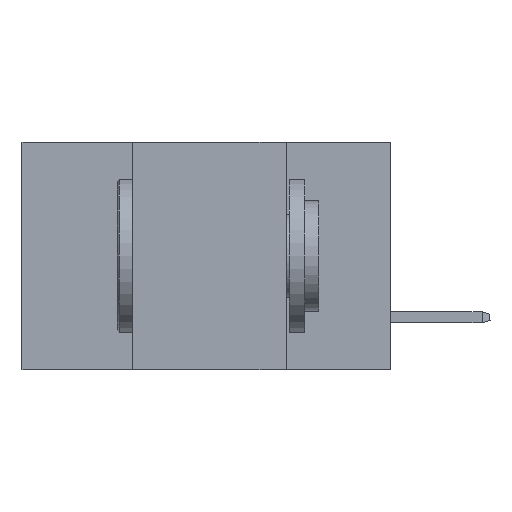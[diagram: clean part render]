
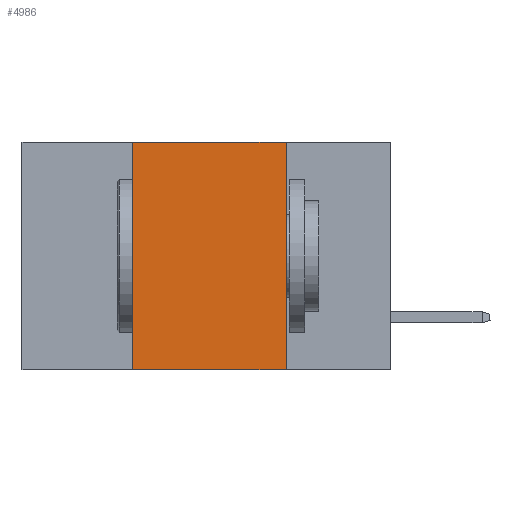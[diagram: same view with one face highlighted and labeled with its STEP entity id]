
A CAD part, left-side view. The second image highlights one B-rep face of the part: STEP entity #4986.
In plain terms, the highlighted planar face has unit normal (-1, 0, 0).
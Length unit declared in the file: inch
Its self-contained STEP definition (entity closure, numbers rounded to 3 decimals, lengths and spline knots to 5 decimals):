
#706 = EDGE_LOOP ( 'NONE', ( #9676, #867, #5534, #11262 ) ) ;
#806 = DIRECTION ( 'NONE',  ( 0., 0., -1. ) ) ;
#867 = ORIENTED_EDGE ( 'NONE', *, *, #1852, .F. ) ;
#901 = CARTESIAN_POINT ( 'NONE',  ( 0., 0.42, 0. ) ) ;
#1179 = CARTESIAN_POINT ( 'NONE',  ( 0., 0.6, -0.37 ) ) ;
#1852 = EDGE_CURVE ( 'NONE', #11017, #5137, #8306, .T. ) ;
#2191 = CARTESIAN_POINT ( 'NONE',  ( 0., 0.17, -0.37 ) ) ;
#2605 = AXIS2_PLACEMENT_3D ( 'NONE', #6672, #11606, #806 ) ;
#2950 = LINE ( 'NONE', #1179, #10446 ) ;
#3140 = CARTESIAN_POINT ( 'NONE',  ( 0., 0.42, 0. ) ) ;
#3214 = CARTESIAN_POINT ( 'NONE',  ( 0., 0.17, 0. ) ) ;
#3239 = EDGE_CURVE ( 'NONE', #8238, #9871, #2950, .T. ) ;
#3992 = VECTOR ( 'NONE', #8603, 39.37008 ) ;
#4698 = PLANE ( 'NONE',  #2605 ) ;
#4986 = ADVANCED_FACE ( 'NONE', ( #9150 ), #4698, .F. ) ;
#5134 = DIRECTION ( 'NONE',  ( 0., 0., 1. ) ) ;
#5137 = VERTEX_POINT ( 'NONE', #3214 ) ;
#5534 = ORIENTED_EDGE ( 'NONE', *, *, #8940, .F. ) ;
#5712 = VECTOR ( 'NONE', #8844, 39.37008 ) ;
#6053 = DIRECTION ( 'NONE',  ( 0., -1., 0. ) ) ;
#6672 = CARTESIAN_POINT ( 'NONE',  ( 0., 0.6, 0. ) ) ;
#6837 = CARTESIAN_POINT ( 'NONE',  ( 0., 0.6, 0. ) ) ;
#6916 = CARTESIAN_POINT ( 'NONE',  ( 0., 0.42, -0.37 ) ) ;
#8238 = VERTEX_POINT ( 'NONE', #6916 ) ;
#8306 = LINE ( 'NONE', #6837, #5712 ) ;
#8603 = DIRECTION ( 'NONE',  ( 0., 0., -1. ) ) ;
#8844 = DIRECTION ( 'NONE',  ( 0., -1., 0. ) ) ;
#8911 = VECTOR ( 'NONE', #5134, 39.37008 ) ;
#8940 = EDGE_CURVE ( 'NONE', #8238, #11017, #10316, .T. ) ;
#9150 = FACE_OUTER_BOUND ( 'NONE', #706, .T. ) ;
#9676 = ORIENTED_EDGE ( 'NONE', *, *, #10718, .F. ) ;
#9871 = VERTEX_POINT ( 'NONE', #2191 ) ;
#10316 = LINE ( 'NONE', #3140, #8911 ) ;
#10446 = VECTOR ( 'NONE', #6053, 39.37008 ) ;
#10718 = EDGE_CURVE ( 'NONE', #5137, #9871, #11846, .T. ) ;
#11017 = VERTEX_POINT ( 'NONE', #901 ) ;
#11262 = ORIENTED_EDGE ( 'NONE', *, *, #3239, .T. ) ;
#11606 = DIRECTION ( 'NONE',  ( 1., 0., 0. ) ) ;
#11846 = LINE ( 'NONE', #12491, #3992 ) ;
#12491 = CARTESIAN_POINT ( 'NONE',  ( 0., 0.17, 0. ) ) ;
